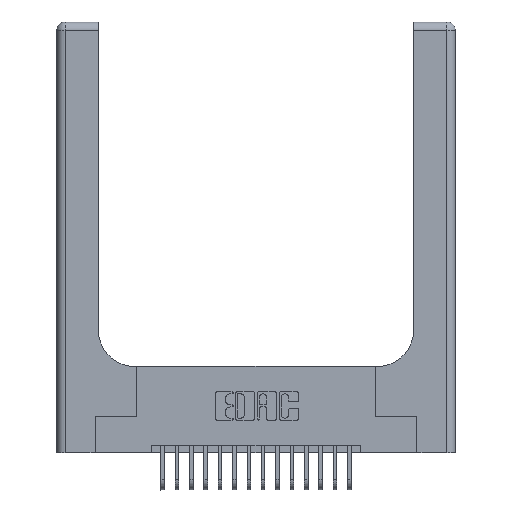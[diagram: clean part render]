
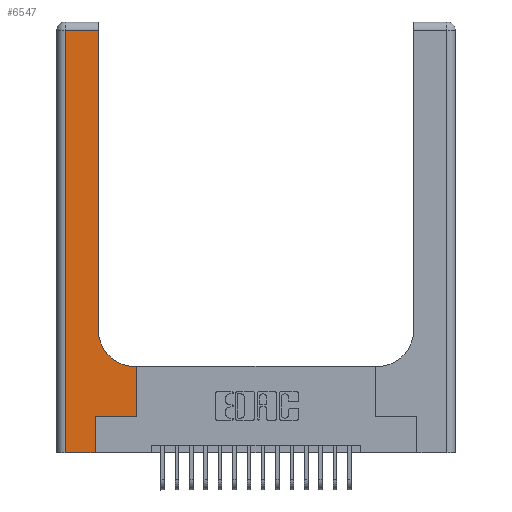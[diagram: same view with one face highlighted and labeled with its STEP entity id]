
A CAD part, top view. The second image highlights one B-rep face of the part: STEP entity #6547.
In plain terms, the highlighted planar face has unit normal (0, 0, 1).
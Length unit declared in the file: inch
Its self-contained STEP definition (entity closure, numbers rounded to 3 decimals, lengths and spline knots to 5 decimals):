
#153 = EDGE_CURVE ( 'NONE', #10148, #12686, #3703, .T. ) ;
#376 = LINE ( 'NONE', #15435, #15558 ) ;
#553 = DIRECTION ( 'NONE',  ( 0., -1., 0. ) ) ;
#918 = LINE ( 'NONE', #10996, #8573 ) ;
#1191 = ORIENTED_EDGE ( 'NONE', *, *, #11742, .T. ) ;
#1194 = CARTESIAN_POINT ( 'NONE',  ( 0.5585, 0.25, 0.37 ) ) ;
#1266 = DIRECTION ( 'NONE',  ( 0., 1., 0. ) ) ;
#1333 = VERTEX_POINT ( 'NONE', #8040 ) ;
#1704 = LINE ( 'NONE', #10089, #5768 ) ;
#1811 = VECTOR ( 'NONE', #4816, 39.37008 ) ;
#1932 = EDGE_LOOP ( 'NONE', ( #14637, #8117, #12531, #12995, #14424, #3356, #11826, #1191, #17221 ) ) ;
#2488 = LINE ( 'NONE', #6645, #6048 ) ;
#2928 = CARTESIAN_POINT ( 'NONE',  ( 0.2915, 0.85, 0.37 ) ) ;
#3027 = CARTESIAN_POINT ( 'NONE',  ( 0.5585, 0.6, 0.37 ) ) ;
#3356 = ORIENTED_EDGE ( 'NONE', *, *, #3803, .T. ) ;
#3703 = CIRCLE ( 'NONE', #13915, 0.25 ) ;
#3803 = EDGE_CURVE ( 'NONE', #16231, #15021, #918, .T. ) ;
#4363 = EDGE_CURVE ( 'NONE', #13926, #6254, #7595, .T. ) ;
#4816 = DIRECTION ( 'NONE',  ( -1., 0., 0. ) ) ;
#5768 = VECTOR ( 'NONE', #17542, 39.37008 ) ;
#5863 = LINE ( 'NONE', #16798, #1811 ) ;
#6048 = VECTOR ( 'NONE', #18595, 39.37008 ) ;
#6254 = VERTEX_POINT ( 'NONE', #11981 ) ;
#6547 = ADVANCED_FACE ( 'NONE', ( #8238 ), #17156, .F. ) ;
#6645 = CARTESIAN_POINT ( 'NONE',  ( 0.2915, 0.6, 0.37 ) ) ;
#6842 = EDGE_CURVE ( 'NONE', #12686, #13290, #7513, .T. ) ;
#7137 = VECTOR ( 'NONE', #1266, 39.37008 ) ;
#7210 = EDGE_CURVE ( 'NONE', #1333, #16231, #1704, .T. ) ;
#7430 = DIRECTION ( 'NONE',  ( 0., 1., 0. ) ) ;
#7513 = LINE ( 'NONE', #16353, #19397 ) ;
#7595 = LINE ( 'NONE', #11227, #11568 ) ;
#8040 = CARTESIAN_POINT ( 'NONE',  ( 0.269, 0., 0.37 ) ) ;
#8117 = ORIENTED_EDGE ( 'NONE', *, *, #14433, .T. ) ;
#8238 = FACE_OUTER_BOUND ( 'NONE', #1932, .T. ) ;
#8573 = VECTOR ( 'NONE', #10926, 39.37008 ) ;
#9730 = DIRECTION ( 'NONE',  ( -1., 0., 0. ) ) ;
#9788 = CARTESIAN_POINT ( 'NONE',  ( 0.5415, 0.6, 0.37 ) ) ;
#10089 = CARTESIAN_POINT ( 'NONE',  ( 0.269, 0., 0.37 ) ) ;
#10148 = VERTEX_POINT ( 'NONE', #9788 ) ;
#10926 = DIRECTION ( 'NONE',  ( 1., 0., 0. ) ) ;
#10996 = CARTESIAN_POINT ( 'NONE',  ( 0.269, 0.25, 0.37 ) ) ;
#11227 = CARTESIAN_POINT ( 'NONE',  ( 0.06, 3., 0.37 ) ) ;
#11514 = VERTEX_POINT ( 'NONE', #3027 ) ;
#11568 = VECTOR ( 'NONE', #553, 39.37008 ) ;
#11742 = EDGE_CURVE ( 'NONE', #11514, #10148, #2488, .T. ) ;
#11826 = ORIENTED_EDGE ( 'NONE', *, *, #18396, .T. ) ;
#11981 = CARTESIAN_POINT ( 'NONE',  ( 0.06, 0., 0.37 ) ) ;
#12531 = ORIENTED_EDGE ( 'NONE', *, *, #4363, .T. ) ;
#12686 = VERTEX_POINT ( 'NONE', #2928 ) ;
#12995 = ORIENTED_EDGE ( 'NONE', *, *, #18607, .T. ) ;
#13290 = VERTEX_POINT ( 'NONE', #19300 ) ;
#13482 = CARTESIAN_POINT ( 'NONE',  ( 0.5585, 0.25, 0.37 ) ) ;
#13493 = DIRECTION ( 'NONE',  ( 1., 0., 0. ) ) ;
#13548 = DIRECTION ( 'NONE',  ( 0., 0., -1. ) ) ;
#13585 = CARTESIAN_POINT ( 'NONE',  ( 0.5415, 0.85, 0.37 ) ) ;
#13915 = AXIS2_PLACEMENT_3D ( 'NONE', #13585, #13548, #13493 ) ;
#13926 = VERTEX_POINT ( 'NONE', #16737 ) ;
#13938 = DIRECTION ( 'NONE',  ( 1., 0., 0. ) ) ;
#14424 = ORIENTED_EDGE ( 'NONE', *, *, #7210, .T. ) ;
#14433 = EDGE_CURVE ( 'NONE', #13290, #13926, #5863, .T. ) ;
#14637 = ORIENTED_EDGE ( 'NONE', *, *, #6842, .T. ) ;
#15021 = VERTEX_POINT ( 'NONE', #13482 ) ;
#15054 = LINE ( 'NONE', #1194, #7137 ) ;
#15197 = AXIS2_PLACEMENT_3D ( 'NONE', #15672, #18677, #9730 ) ;
#15435 = CARTESIAN_POINT ( 'NONE',  ( 0., 0., 0.37 ) ) ;
#15558 = VECTOR ( 'NONE', #13938, 39.37008 ) ;
#15672 = CARTESIAN_POINT ( 'NONE',  ( 0., 3., 0.37 ) ) ;
#16231 = VERTEX_POINT ( 'NONE', #16678 ) ;
#16353 = CARTESIAN_POINT ( 'NONE',  ( 0.2915, 3., 0.37 ) ) ;
#16678 = CARTESIAN_POINT ( 'NONE',  ( 0.269, 0.25, 0.37 ) ) ;
#16737 = CARTESIAN_POINT ( 'NONE',  ( 0.06, 2.94, 0.37 ) ) ;
#16798 = CARTESIAN_POINT ( 'NONE',  ( 0., 2.94, 0.37 ) ) ;
#17156 = PLANE ( 'NONE',  #15197 ) ;
#17221 = ORIENTED_EDGE ( 'NONE', *, *, #153, .T. ) ;
#17542 = DIRECTION ( 'NONE',  ( 0., 1., 0. ) ) ;
#18396 = EDGE_CURVE ( 'NONE', #15021, #11514, #15054, .T. ) ;
#18595 = DIRECTION ( 'NONE',  ( -1., 0., 0. ) ) ;
#18607 = EDGE_CURVE ( 'NONE', #6254, #1333, #376, .T. ) ;
#18677 = DIRECTION ( 'NONE',  ( 0., 0., -1. ) ) ;
#19300 = CARTESIAN_POINT ( 'NONE',  ( 0.2915, 2.94, 0.37 ) ) ;
#19397 = VECTOR ( 'NONE', #7430, 39.37008 ) ;
